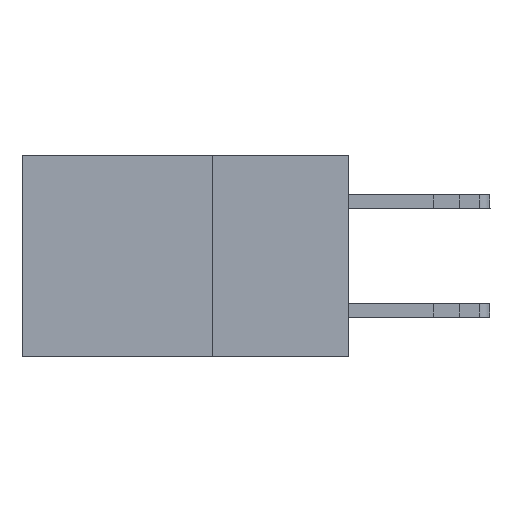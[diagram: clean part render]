
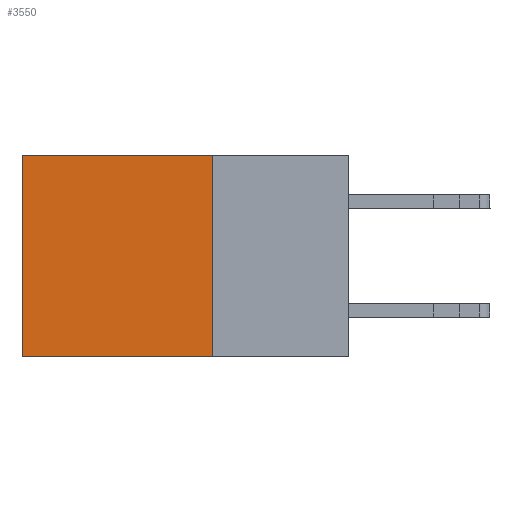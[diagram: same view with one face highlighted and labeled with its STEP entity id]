
A CAD part, left-side view. The second image highlights one B-rep face of the part: STEP entity #3550.
In plain terms, the highlighted planar face has unit normal (-1, 0, 0).
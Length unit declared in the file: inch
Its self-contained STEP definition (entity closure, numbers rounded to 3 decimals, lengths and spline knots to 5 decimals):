
#135 = CARTESIAN_POINT ( 'NONE',  ( 0.298, 0.25, 0. ) ) ;
#353 = CARTESIAN_POINT ( 'NONE',  ( 0.298, 0.25, 0. ) ) ;
#373 = DIRECTION ( 'NONE',  ( 0., 1., 0. ) ) ;
#994 = EDGE_CURVE ( 'NONE', #11423, #2095, #6468, .T. ) ;
#1671 = LINE ( 'NONE', #6281, #8340 ) ;
#1889 = ORIENTED_EDGE ( 'NONE', *, *, #994, .T. ) ;
#2095 = VERTEX_POINT ( 'NONE', #3340 ) ;
#2313 = FACE_OUTER_BOUND ( 'NONE', #11241, .T. ) ;
#3267 = CARTESIAN_POINT ( 'NONE',  ( 0.298, 0.25, -0.37 ) ) ;
#3340 = CARTESIAN_POINT ( 'NONE',  ( 0.298, 0.6, -0.37 ) ) ;
#3550 = ADVANCED_FACE ( 'NONE', ( #2313 ), #4645, .F. ) ;
#4114 = ORIENTED_EDGE ( 'NONE', *, *, #13015, .T. ) ;
#4134 = DIRECTION ( 'NONE',  ( 0., 0., -1. ) ) ;
#4349 = VERTEX_POINT ( 'NONE', #3267 ) ;
#4449 = EDGE_CURVE ( 'NONE', #11924, #4349, #10527, .T. ) ;
#4473 = VECTOR ( 'NONE', #9767, 39.37008 ) ;
#4645 = PLANE ( 'NONE',  #6296 ) ;
#4660 = CARTESIAN_POINT ( 'NONE',  ( 0.298, 0.25, 0. ) ) ;
#4789 = CARTESIAN_POINT ( 'NONE',  ( 0.298, 0.25, 0. ) ) ;
#6075 = DIRECTION ( 'NONE',  ( 1., 0., 0. ) ) ;
#6281 = CARTESIAN_POINT ( 'NONE',  ( 0.298, 0.25, -0.37 ) ) ;
#6296 = AXIS2_PLACEMENT_3D ( 'NONE', #4789, #6075, #8430 ) ;
#6389 = CARTESIAN_POINT ( 'NONE',  ( 0.298, 0.6, 0. ) ) ;
#6468 = LINE ( 'NONE', #6389, #7168 ) ;
#7168 = VECTOR ( 'NONE', #4134, 39.37008 ) ;
#8340 = VECTOR ( 'NONE', #373, 39.37008 ) ;
#8361 = ORIENTED_EDGE ( 'NONE', *, *, #4449, .F. ) ;
#8430 = DIRECTION ( 'NONE',  ( 0., 0., -1. ) ) ;
#9767 = DIRECTION ( 'NONE',  ( 0., 1., 0. ) ) ;
#10454 = DIRECTION ( 'NONE',  ( 0., 0., -1. ) ) ;
#10527 = LINE ( 'NONE', #135, #14352 ) ;
#10744 = CARTESIAN_POINT ( 'NONE',  ( 0.298, 0.6, 0. ) ) ;
#11241 = EDGE_LOOP ( 'NONE', ( #1889, #13190, #8361, #4114 ) ) ;
#11423 = VERTEX_POINT ( 'NONE', #10744 ) ;
#11924 = VERTEX_POINT ( 'NONE', #4660 ) ;
#12487 = EDGE_CURVE ( 'NONE', #4349, #2095, #1671, .T. ) ;
#13015 = EDGE_CURVE ( 'NONE', #11924, #11423, #14382, .T. ) ;
#13190 = ORIENTED_EDGE ( 'NONE', *, *, #12487, .F. ) ;
#14352 = VECTOR ( 'NONE', #10454, 39.37008 ) ;
#14382 = LINE ( 'NONE', #353, #4473 ) ;
